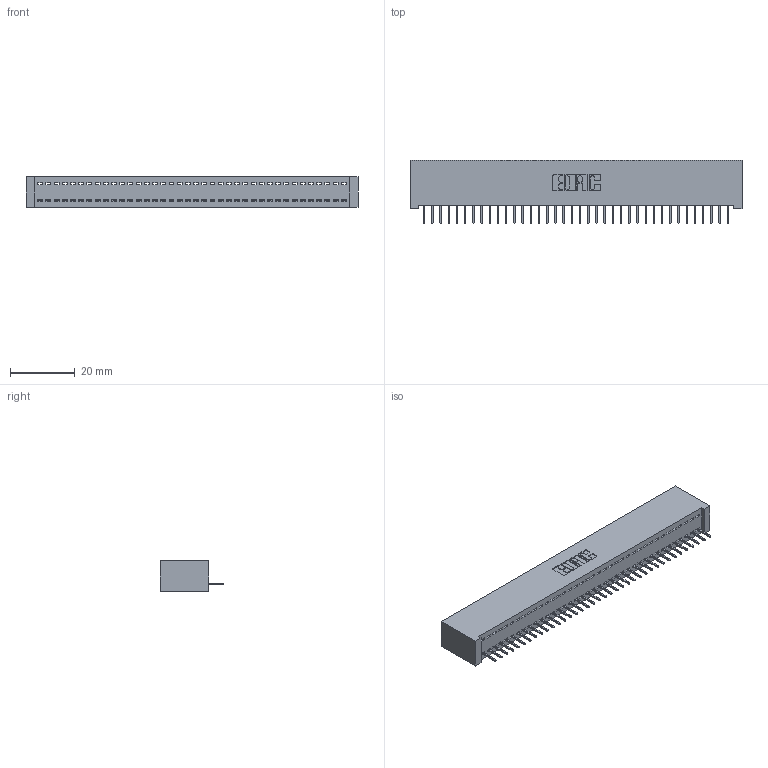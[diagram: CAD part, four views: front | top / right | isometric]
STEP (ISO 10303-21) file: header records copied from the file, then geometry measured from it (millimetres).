
FILE_DESCRIPTION (( 'STEP AP203' ), '1' );
FILE_NAME ('392-038-524-101.STEP', '2018-08-16T05:06:54', ( '' ), ( '' ), 'SwSTEP 2.0', 'SolidWorks 2016', '' );
FILE_SCHEMA (( 'CONFIG_CONTROL_DESIGN' ));
Length unit declared in the file: inch
Products named in the file (3): 342 Part_Lugless; 345-292-001_345-293-124; 392-038-524-101
Assembly tree (39 placements, depth 2):
  392-038-524-101
    342 Part_Lugless
    345-292-001_345-293-124  x38
Bounding box: 102.77 x 19.69 x 9.4 mm (x, y, z)
Volume: 9254.9 mm3; surface area: 13372.7 mm2
Topology: 39 solids, 39 shells, 2458 faces, 7115 edges, 4590 vertices
Faces by surface type: plane 1886, cylinder 572
Entity records: 23413 total; most frequent: CARTESIAN_POINT 4044, ORIENTED_EDGE 4018, DIRECTION 3413, EDGE_CURVE 2009, VECTOR 1893, LINE 1893, VERTEX_POINT 1334, AXIS2_PLACEMENT_3D 760
